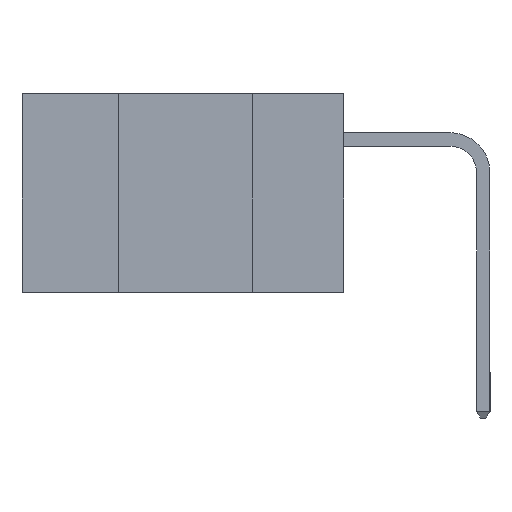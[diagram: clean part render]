
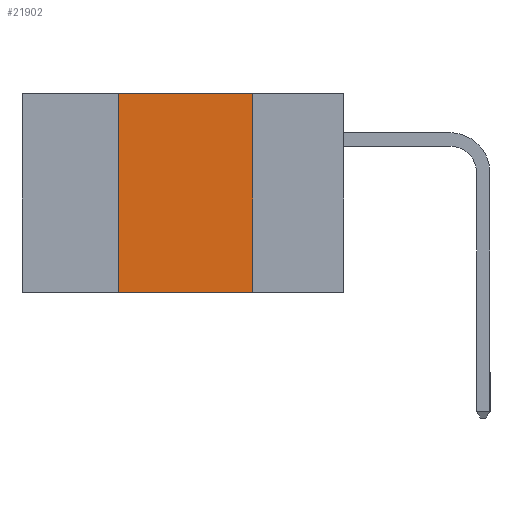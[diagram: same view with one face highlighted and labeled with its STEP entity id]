
A CAD part, left-side view. The second image highlights one B-rep face of the part: STEP entity #21902.
In plain terms, the highlighted planar face has unit normal (-1, 0, 0).
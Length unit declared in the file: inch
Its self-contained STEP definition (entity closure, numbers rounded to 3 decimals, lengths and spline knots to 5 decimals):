
#1069 = DIRECTION ( 'NONE',  ( 0., 0., -1. ) ) ;
#1751 = EDGE_CURVE ( 'NONE', #6768, #3488, #23904, .T. ) ;
#2631 = CARTESIAN_POINT ( 'NONE',  ( 0., 0.6, 0. ) ) ;
#2927 = CARTESIAN_POINT ( 'NONE',  ( 0., 0.17, 0. ) ) ;
#3488 = VERTEX_POINT ( 'NONE', #14872 ) ;
#3748 = CARTESIAN_POINT ( 'NONE',  ( 0., 0.6, 0. ) ) ;
#4635 = ORIENTED_EDGE ( 'NONE', *, *, #6507, .F. ) ;
#5574 = DIRECTION ( 'NONE',  ( 0., -1., 0. ) ) ;
#6045 = EDGE_CURVE ( 'NONE', #17258, #6768, #10166, .T. ) ;
#6507 = EDGE_CURVE ( 'NONE', #13160, #17258, #15784, .T. ) ;
#6768 = VERTEX_POINT ( 'NONE', #22319 ) ;
#7011 = VECTOR ( 'NONE', #5574, 39.37008 ) ;
#7684 = EDGE_LOOP ( 'NONE', ( #18026, #12245, #4635, #16009 ) ) ;
#9368 = DIRECTION ( 'NONE',  ( 0., -1., 0. ) ) ;
#10166 = LINE ( 'NONE', #3748, #7011 ) ;
#10602 = DIRECTION ( 'NONE',  ( 1., 0., 0. ) ) ;
#11435 = VECTOR ( 'NONE', #1069, 39.37008 ) ;
#11510 = DIRECTION ( 'NONE',  ( 0., 0., 1. ) ) ;
#12245 = ORIENTED_EDGE ( 'NONE', *, *, #6045, .F. ) ;
#12544 = EDGE_CURVE ( 'NONE', #13160, #3488, #25555, .T. ) ;
#12590 = DIRECTION ( 'NONE',  ( 0., 0., -1. ) ) ;
#12990 = VECTOR ( 'NONE', #11510, 39.37008 ) ;
#13160 = VERTEX_POINT ( 'NONE', #21731 ) ;
#14626 = PLANE ( 'NONE',  #24714 ) ;
#14872 = CARTESIAN_POINT ( 'NONE',  ( 0., 0.17, -0.37 ) ) ;
#15420 = CARTESIAN_POINT ( 'NONE',  ( 0., 0.42, 0. ) ) ;
#15784 = LINE ( 'NONE', #23435, #12990 ) ;
#16009 = ORIENTED_EDGE ( 'NONE', *, *, #12544, .T. ) ;
#17258 = VERTEX_POINT ( 'NONE', #15420 ) ;
#18026 = ORIENTED_EDGE ( 'NONE', *, *, #1751, .F. ) ;
#18369 = VECTOR ( 'NONE', #9368, 39.37008 ) ;
#21334 = CARTESIAN_POINT ( 'NONE',  ( 0., 0.6, -0.37 ) ) ;
#21731 = CARTESIAN_POINT ( 'NONE',  ( 0., 0.42, -0.37 ) ) ;
#21902 = ADVANCED_FACE ( 'NONE', ( #23294 ), #14626, .F. ) ;
#22319 = CARTESIAN_POINT ( 'NONE',  ( 0., 0.17, 0. ) ) ;
#23294 = FACE_OUTER_BOUND ( 'NONE', #7684, .T. ) ;
#23435 = CARTESIAN_POINT ( 'NONE',  ( 0., 0.42, 0. ) ) ;
#23904 = LINE ( 'NONE', #2927, #11435 ) ;
#24714 = AXIS2_PLACEMENT_3D ( 'NONE', #2631, #10602, #12590 ) ;
#25555 = LINE ( 'NONE', #21334, #18369 ) ;
